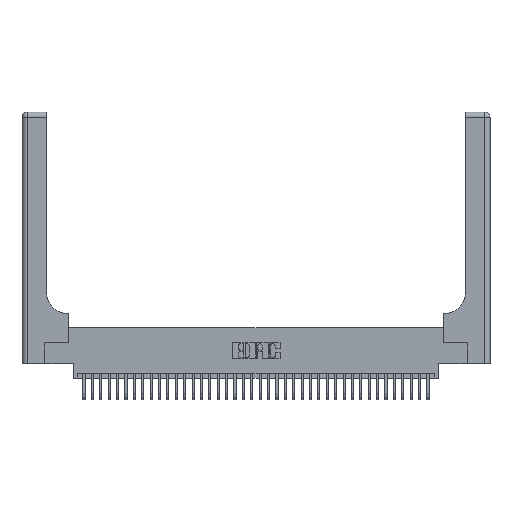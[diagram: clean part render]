
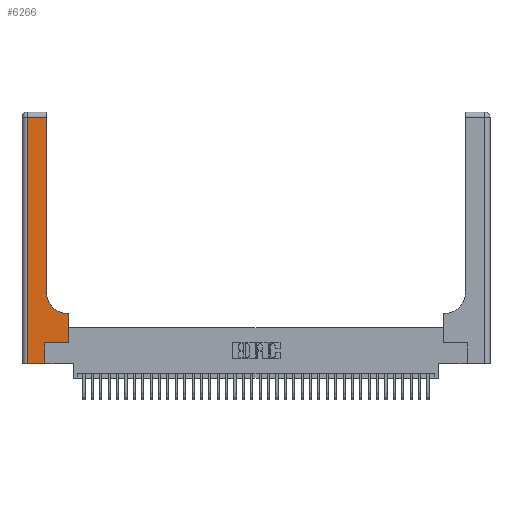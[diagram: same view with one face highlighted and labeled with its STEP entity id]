
A CAD part, top view. The second image highlights one B-rep face of the part: STEP entity #6266.
In plain terms, the highlighted planar face has unit normal (0, 0, 1).
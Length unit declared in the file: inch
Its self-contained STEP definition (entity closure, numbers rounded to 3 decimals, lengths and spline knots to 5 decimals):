
#799 = ORIENTED_EDGE ( 'NONE', *, *, #22688, .T. ) ;
#874 = VERTEX_POINT ( 'NONE', #33500 ) ;
#1614 = LINE ( 'NONE', #33099, #36034 ) ;
#1700 = ORIENTED_EDGE ( 'NONE', *, *, #33766, .T. ) ;
#1812 = CIRCLE ( 'NONE', #5447, 0.25 ) ;
#2189 = EDGE_CURVE ( 'NONE', #21268, #9999, #5686, .T. ) ;
#2364 = LINE ( 'NONE', #24615, #9869 ) ;
#3018 = CARTESIAN_POINT ( 'NONE',  ( 0., 2.94, 0.37 ) ) ;
#3821 = PLANE ( 'NONE',  #23435 ) ;
#4930 = VERTEX_POINT ( 'NONE', #20359 ) ;
#5051 = CARTESIAN_POINT ( 'NONE',  ( 0.06, 0., 0.37 ) ) ;
#5229 = EDGE_CURVE ( 'NONE', #6553, #34131, #2364, .T. ) ;
#5354 = ORIENTED_EDGE ( 'NONE', *, *, #24939, .T. ) ;
#5447 = AXIS2_PLACEMENT_3D ( 'NONE', #23865, #6725, #26793 ) ;
#5550 = LINE ( 'NONE', #21314, #19822 ) ;
#5686 = LINE ( 'NONE', #28715, #35220 ) ;
#6266 = ADVANCED_FACE ( 'NONE', ( #23266 ), #3821, .F. ) ;
#6553 = VERTEX_POINT ( 'NONE', #5051 ) ;
#6725 = DIRECTION ( 'NONE',  ( 0., 0., -1. ) ) ;
#7438 = DIRECTION ( 'NONE',  ( 1., 0., 0. ) ) ;
#7446 = ORIENTED_EDGE ( 'NONE', *, *, #8571, .T. ) ;
#8503 = EDGE_CURVE ( 'NONE', #4930, #21268, #1614, .T. ) ;
#8571 = EDGE_CURVE ( 'NONE', #34131, #11894, #25779, .T. ) ;
#8712 = CARTESIAN_POINT ( 'NONE',  ( 0.06, 2.94, 0.37 ) ) ;
#8985 = VECTOR ( 'NONE', #31692, 39.37008 ) ;
#9206 = EDGE_LOOP ( 'NONE', ( #1700, #36997, #5354, #33115, #7446, #12354, #9305, #31346, #799 ) ) ;
#9305 = ORIENTED_EDGE ( 'NONE', *, *, #8503, .T. ) ;
#9501 = CARTESIAN_POINT ( 'NONE',  ( 0., 3., 0.37 ) ) ;
#9869 = VECTOR ( 'NONE', #7438, 39.37008 ) ;
#9892 = DIRECTION ( 'NONE',  ( 1., 0., 0. ) ) ;
#9999 = VERTEX_POINT ( 'NONE', #14418 ) ;
#10618 = DIRECTION ( 'NONE',  ( 0., 1., 0. ) ) ;
#11795 = CARTESIAN_POINT ( 'NONE',  ( 0.269, 0.25, 0.37 ) ) ;
#11797 = CARTESIAN_POINT ( 'NONE',  ( 0.5585, 0.6, 0.37 ) ) ;
#11894 = VERTEX_POINT ( 'NONE', #11795 ) ;
#12354 = ORIENTED_EDGE ( 'NONE', *, *, #19639, .T. ) ;
#12388 = DIRECTION ( 'NONE',  ( -1., 0., 0. ) ) ;
#13264 = DIRECTION ( 'NONE',  ( 0., 1., 0. ) ) ;
#14418 = CARTESIAN_POINT ( 'NONE',  ( 0.5415, 0.6, 0.37 ) ) ;
#16584 = LINE ( 'NONE', #3018, #8985 ) ;
#16922 = EDGE_CURVE ( 'NONE', #32879, #22486, #16584, .T. ) ;
#18076 = VECTOR ( 'NONE', #10618, 39.37008 ) ;
#19639 = EDGE_CURVE ( 'NONE', #11894, #4930, #5550, .T. ) ;
#19822 = VECTOR ( 'NONE', #9892, 39.37008 ) ;
#20359 = CARTESIAN_POINT ( 'NONE',  ( 0.5585, 0.25, 0.37 ) ) ;
#21268 = VERTEX_POINT ( 'NONE', #11797 ) ;
#21314 = CARTESIAN_POINT ( 'NONE',  ( 0.269, 0.25, 0.37 ) ) ;
#22486 = VERTEX_POINT ( 'NONE', #8712 ) ;
#22611 = DIRECTION ( 'NONE',  ( 0., -1., 0. ) ) ;
#22688 = EDGE_CURVE ( 'NONE', #9999, #874, #1812, .T. ) ;
#22806 = VECTOR ( 'NONE', #13264, 39.37008 ) ;
#23266 = FACE_OUTER_BOUND ( 'NONE', #9206, .T. ) ;
#23435 = AXIS2_PLACEMENT_3D ( 'NONE', #9501, #29654, #12388 ) ;
#23628 = CARTESIAN_POINT ( 'NONE',  ( 0.2915, 2.94, 0.37 ) ) ;
#23865 = CARTESIAN_POINT ( 'NONE',  ( 0.5415, 0.85, 0.37 ) ) ;
#24615 = CARTESIAN_POINT ( 'NONE',  ( 0., 0., 0.37 ) ) ;
#24939 = EDGE_CURVE ( 'NONE', #22486, #6553, #28816, .T. ) ;
#25779 = LINE ( 'NONE', #33469, #18076 ) ;
#26793 = DIRECTION ( 'NONE',  ( 1., 0., 0. ) ) ;
#28715 = CARTESIAN_POINT ( 'NONE',  ( 0.2915, 0.6, 0.37 ) ) ;
#28816 = LINE ( 'NONE', #36732, #36321 ) ;
#29600 = LINE ( 'NONE', #30524, #22806 ) ;
#29654 = DIRECTION ( 'NONE',  ( 0., 0., -1. ) ) ;
#30524 = CARTESIAN_POINT ( 'NONE',  ( 0.2915, 3., 0.37 ) ) ;
#31346 = ORIENTED_EDGE ( 'NONE', *, *, #2189, .T. ) ;
#31692 = DIRECTION ( 'NONE',  ( -1., 0., 0. ) ) ;
#32879 = VERTEX_POINT ( 'NONE', #23628 ) ;
#33099 = CARTESIAN_POINT ( 'NONE',  ( 0.5585, 0.25, 0.37 ) ) ;
#33115 = ORIENTED_EDGE ( 'NONE', *, *, #5229, .T. ) ;
#33469 = CARTESIAN_POINT ( 'NONE',  ( 0.269, 0., 0.37 ) ) ;
#33500 = CARTESIAN_POINT ( 'NONE',  ( 0.2915, 0.85, 0.37 ) ) ;
#33766 = EDGE_CURVE ( 'NONE', #874, #32879, #29600, .T. ) ;
#34131 = VERTEX_POINT ( 'NONE', #35546 ) ;
#34415 = DIRECTION ( 'NONE',  ( -1., 0., 0. ) ) ;
#35220 = VECTOR ( 'NONE', #34415, 39.37008 ) ;
#35546 = CARTESIAN_POINT ( 'NONE',  ( 0.269, 0., 0.37 ) ) ;
#35929 = DIRECTION ( 'NONE',  ( 0., 1., 0. ) ) ;
#36034 = VECTOR ( 'NONE', #35929, 39.37008 ) ;
#36321 = VECTOR ( 'NONE', #22611, 39.37008 ) ;
#36732 = CARTESIAN_POINT ( 'NONE',  ( 0.06, 3., 0.37 ) ) ;
#36997 = ORIENTED_EDGE ( 'NONE', *, *, #16922, .T. ) ;
